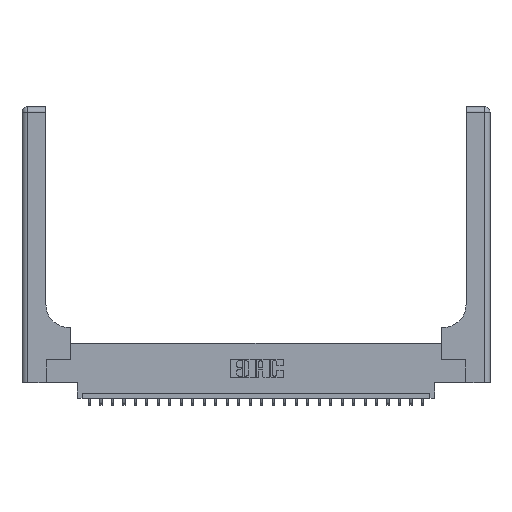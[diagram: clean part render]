
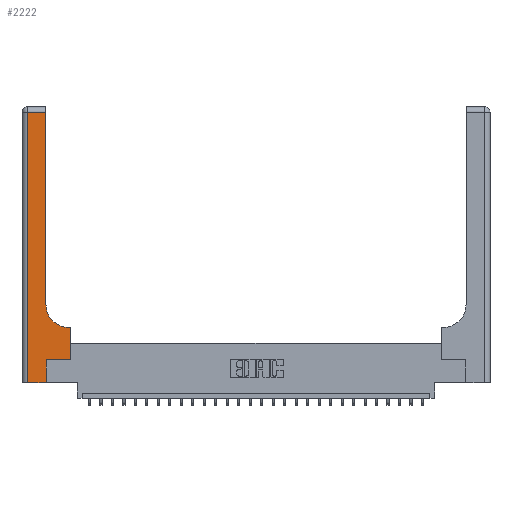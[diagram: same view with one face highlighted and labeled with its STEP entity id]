
A CAD part, top view. The second image highlights one B-rep face of the part: STEP entity #2222.
In plain terms, the highlighted planar face has unit normal (0, 0, 1).
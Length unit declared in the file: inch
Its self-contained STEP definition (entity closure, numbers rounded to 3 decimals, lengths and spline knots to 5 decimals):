
#313 = DIRECTION ( 'NONE',  ( 0., 1., 0. ) ) ;
#564 = CARTESIAN_POINT ( 'NONE',  ( 0.26, 0.85, 0.37 ) ) ;
#759 = CARTESIAN_POINT ( 'NONE',  ( 0.06, 2.94, 0.37 ) ) ;
#1267 = DIRECTION ( 'NONE',  ( -1., 0., 0. ) ) ;
#1325 = ORIENTED_EDGE ( 'NONE', *, *, #9548, .T. ) ;
#1452 = LINE ( 'NONE', #19507, #18203 ) ;
#2222 = ADVANCED_FACE ( 'NONE', ( #6949 ), #5364, .F. ) ;
#2527 = VECTOR ( 'NONE', #25270, 39.37008 ) ;
#2973 = CARTESIAN_POINT ( 'NONE',  ( 0., 3., 0.37 ) ) ;
#3038 = ORIENTED_EDGE ( 'NONE', *, *, #9277, .T. ) ;
#3851 = EDGE_LOOP ( 'NONE', ( #25137, #17676, #9323, #14548, #12940, #1325, #3038, #15728, #11733 ) ) ;
#3907 = CARTESIAN_POINT ( 'NONE',  ( 0.06, 3., 0.37 ) ) ;
#4236 = CARTESIAN_POINT ( 'NONE',  ( 0.528, 0.25, 0.37 ) ) ;
#4801 = DIRECTION ( 'NONE',  ( 1., 0., 0. ) ) ;
#4874 = CARTESIAN_POINT ( 'NONE',  ( 0.06, 0., 0.37 ) ) ;
#5364 = PLANE ( 'NONE',  #13156 ) ;
#5726 = CARTESIAN_POINT ( 'NONE',  ( 0.265, 0.25, 0.37 ) ) ;
#5795 = EDGE_CURVE ( 'NONE', #17412, #6091, #1452, .T. ) ;
#6091 = VERTEX_POINT ( 'NONE', #759 ) ;
#6374 = CARTESIAN_POINT ( 'NONE',  ( 0.265, 0.25, 0.37 ) ) ;
#6685 = CARTESIAN_POINT ( 'NONE',  ( 0.26, 2.94, 0.37 ) ) ;
#6949 = FACE_OUTER_BOUND ( 'NONE', #3851, .T. ) ;
#7709 = VECTOR ( 'NONE', #4801, 39.37008 ) ;
#8312 = CARTESIAN_POINT ( 'NONE',  ( 0.51, 0.85, 0.37 ) ) ;
#8485 = VERTEX_POINT ( 'NONE', #5726 ) ;
#8574 = CIRCLE ( 'NONE', #9411, 0.25 ) ;
#8785 = CARTESIAN_POINT ( 'NONE',  ( 0.26, 0.6, 0.37 ) ) ;
#8872 = LINE ( 'NONE', #6374, #7709 ) ;
#9127 = VERTEX_POINT ( 'NONE', #4874 ) ;
#9256 = VECTOR ( 'NONE', #22127, 39.37008 ) ;
#9277 = EDGE_CURVE ( 'NONE', #12494, #11392, #22465, .T. ) ;
#9323 = ORIENTED_EDGE ( 'NONE', *, *, #20418, .T. ) ;
#9411 = AXIS2_PLACEMENT_3D ( 'NONE', #8312, #9775, #16217 ) ;
#9548 = EDGE_CURVE ( 'NONE', #8485, #12494, #8872, .T. ) ;
#9775 = DIRECTION ( 'NONE',  ( 0., 0., -1. ) ) ;
#10878 = EDGE_CURVE ( 'NONE', #14774, #8485, #24575, .T. ) ;
#11392 = VERTEX_POINT ( 'NONE', #17546 ) ;
#11733 = ORIENTED_EDGE ( 'NONE', *, *, #21134, .T. ) ;
#11928 = VECTOR ( 'NONE', #20363, 39.37008 ) ;
#12494 = VERTEX_POINT ( 'NONE', #4236 ) ;
#12810 = VECTOR ( 'NONE', #22595, 39.37008 ) ;
#12940 = ORIENTED_EDGE ( 'NONE', *, *, #10878, .T. ) ;
#13156 = AXIS2_PLACEMENT_3D ( 'NONE', #2973, #22898, #1267 ) ;
#14127 = DIRECTION ( 'NONE',  ( -1., 0., 0. ) ) ;
#14164 = VERTEX_POINT ( 'NONE', #21643 ) ;
#14548 = ORIENTED_EDGE ( 'NONE', *, *, #17189, .T. ) ;
#14774 = VERTEX_POINT ( 'NONE', #25156 ) ;
#15684 = VECTOR ( 'NONE', #19988, 39.37008 ) ;
#15728 = ORIENTED_EDGE ( 'NONE', *, *, #17557, .T. ) ;
#16158 = LINE ( 'NONE', #3907, #15684 ) ;
#16217 = DIRECTION ( 'NONE',  ( 1., 0., 0. ) ) ;
#16524 = CARTESIAN_POINT ( 'NONE',  ( 0.528, 0.25, 0.37 ) ) ;
#16729 = VERTEX_POINT ( 'NONE', #564 ) ;
#17189 = EDGE_CURVE ( 'NONE', #9127, #14774, #18161, .T. ) ;
#17412 = VERTEX_POINT ( 'NONE', #6685 ) ;
#17546 = CARTESIAN_POINT ( 'NONE',  ( 0.528, 0.6, 0.37 ) ) ;
#17557 = EDGE_CURVE ( 'NONE', #11392, #14164, #18805, .T. ) ;
#17676 = ORIENTED_EDGE ( 'NONE', *, *, #5795, .T. ) ;
#18161 = LINE ( 'NONE', #22378, #9256 ) ;
#18203 = VECTOR ( 'NONE', #14127, 39.37008 ) ;
#18627 = CARTESIAN_POINT ( 'NONE',  ( 0.265, 0., 0.37 ) ) ;
#18805 = LINE ( 'NONE', #8785, #2527 ) ;
#19002 = CARTESIAN_POINT ( 'NONE',  ( 0.26, 3., 0.37 ) ) ;
#19507 = CARTESIAN_POINT ( 'NONE',  ( 0., 2.94, 0.37 ) ) ;
#19988 = DIRECTION ( 'NONE',  ( 0., -1., 0. ) ) ;
#20363 = DIRECTION ( 'NONE',  ( 0., 1., 0. ) ) ;
#20418 = EDGE_CURVE ( 'NONE', #6091, #9127, #16158, .T. ) ;
#20890 = EDGE_CURVE ( 'NONE', #16729, #17412, #21116, .T. ) ;
#21116 = LINE ( 'NONE', #19002, #11928 ) ;
#21134 = EDGE_CURVE ( 'NONE', #14164, #16729, #8574, .T. ) ;
#21592 = VECTOR ( 'NONE', #313, 39.37008 ) ;
#21643 = CARTESIAN_POINT ( 'NONE',  ( 0.51, 0.6, 0.37 ) ) ;
#22127 = DIRECTION ( 'NONE',  ( 1., 0., 0. ) ) ;
#22378 = CARTESIAN_POINT ( 'NONE',  ( 0., 0., 0.37 ) ) ;
#22465 = LINE ( 'NONE', #16524, #21592 ) ;
#22595 = DIRECTION ( 'NONE',  ( 0., 1., 0. ) ) ;
#22898 = DIRECTION ( 'NONE',  ( 0., 0., -1. ) ) ;
#24575 = LINE ( 'NONE', #18627, #12810 ) ;
#25137 = ORIENTED_EDGE ( 'NONE', *, *, #20890, .T. ) ;
#25156 = CARTESIAN_POINT ( 'NONE',  ( 0.265, 0., 0.37 ) ) ;
#25270 = DIRECTION ( 'NONE',  ( -1., 0., 0. ) ) ;
